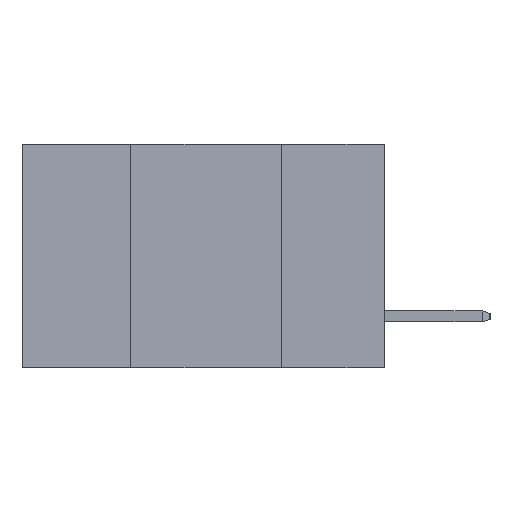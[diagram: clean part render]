
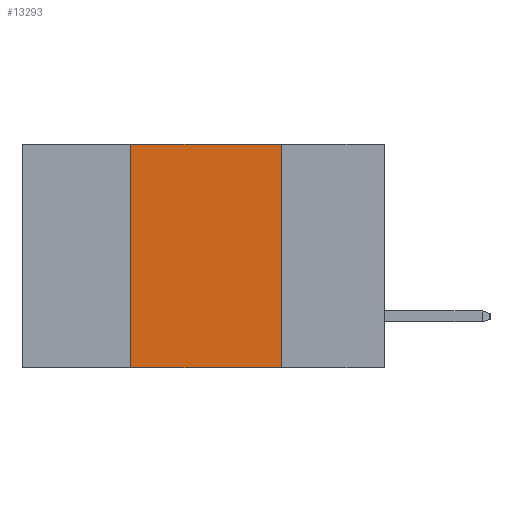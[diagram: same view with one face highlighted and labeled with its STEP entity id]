
A CAD part, left-side view. The second image highlights one B-rep face of the part: STEP entity #13293.
In plain terms, the highlighted planar face has unit normal (-1, 0, 0).
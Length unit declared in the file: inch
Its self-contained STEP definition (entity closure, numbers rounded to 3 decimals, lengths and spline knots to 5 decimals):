
#668 = DIRECTION ( 'NONE',  ( 0., -1., 0. ) ) ;
#819 = LINE ( 'NONE', #11643, #10655 ) ;
#1173 = VECTOR ( 'NONE', #668, 39.37008 ) ;
#1330 = ORIENTED_EDGE ( 'NONE', *, *, #18826, .F. ) ;
#1614 = PLANE ( 'NONE',  #25293 ) ;
#3563 = EDGE_CURVE ( 'NONE', #12631, #17241, #11431, .T. ) ;
#5593 = DIRECTION ( 'NONE',  ( 0., 0., -1. ) ) ;
#5662 = CARTESIAN_POINT ( 'NONE',  ( 0., 0.17, -0.37 ) ) ;
#6245 = VECTOR ( 'NONE', #7175, 39.37008 ) ;
#7017 = LINE ( 'NONE', #24068, #1173 ) ;
#7175 = DIRECTION ( 'NONE',  ( 0., 0., -1. ) ) ;
#7405 = VECTOR ( 'NONE', #10489, 39.37008 ) ;
#7439 = CARTESIAN_POINT ( 'NONE',  ( 0., 0.17, 0. ) ) ;
#9391 = FACE_OUTER_BOUND ( 'NONE', #11816, .T. ) ;
#10489 = DIRECTION ( 'NONE',  ( 0., -1., 0. ) ) ;
#10585 = EDGE_CURVE ( 'NONE', #13446, #17241, #7017, .T. ) ;
#10655 = VECTOR ( 'NONE', #13563, 39.37008 ) ;
#11431 = LINE ( 'NONE', #7439, #6245 ) ;
#11643 = CARTESIAN_POINT ( 'NONE',  ( 0., 0.42, 0. ) ) ;
#11816 = EDGE_LOOP ( 'NONE', ( #19750, #1330, #22768, #22487 ) ) ;
#12631 = VERTEX_POINT ( 'NONE', #24642 ) ;
#13293 = ADVANCED_FACE ( 'NONE', ( #9391 ), #1614, .F. ) ;
#13446 = VERTEX_POINT ( 'NONE', #15740 ) ;
#13563 = DIRECTION ( 'NONE',  ( 0., 0., 1. ) ) ;
#15218 = CARTESIAN_POINT ( 'NONE',  ( 0., 0.6, 0. ) ) ;
#15740 = CARTESIAN_POINT ( 'NONE',  ( 0., 0.42, -0.37 ) ) ;
#17241 = VERTEX_POINT ( 'NONE', #5662 ) ;
#17249 = DIRECTION ( 'NONE',  ( 1., 0., 0. ) ) ;
#18826 = EDGE_CURVE ( 'NONE', #22372, #12631, #22984, .T. ) ;
#19750 = ORIENTED_EDGE ( 'NONE', *, *, #3563, .F. ) ;
#20238 = CARTESIAN_POINT ( 'NONE',  ( 0., 0.6, 0. ) ) ;
#22372 = VERTEX_POINT ( 'NONE', #25124 ) ;
#22487 = ORIENTED_EDGE ( 'NONE', *, *, #10585, .T. ) ;
#22768 = ORIENTED_EDGE ( 'NONE', *, *, #23641, .F. ) ;
#22984 = LINE ( 'NONE', #20238, #7405 ) ;
#23641 = EDGE_CURVE ( 'NONE', #13446, #22372, #819, .T. ) ;
#24068 = CARTESIAN_POINT ( 'NONE',  ( 0., 0.6, -0.37 ) ) ;
#24642 = CARTESIAN_POINT ( 'NONE',  ( 0., 0.17, 0. ) ) ;
#25124 = CARTESIAN_POINT ( 'NONE',  ( 0., 0.42, 0. ) ) ;
#25293 = AXIS2_PLACEMENT_3D ( 'NONE', #15218, #17249, #5593 ) ;
